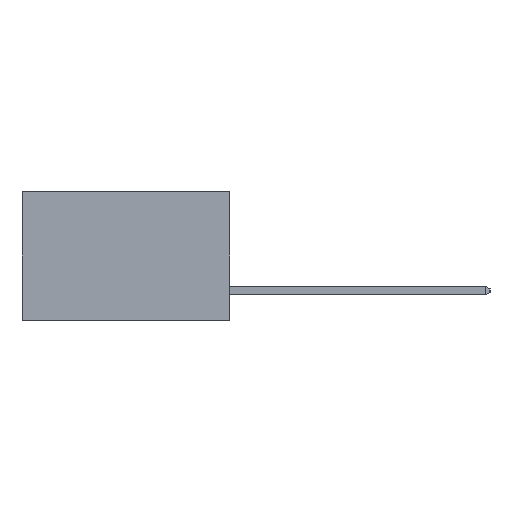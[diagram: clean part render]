
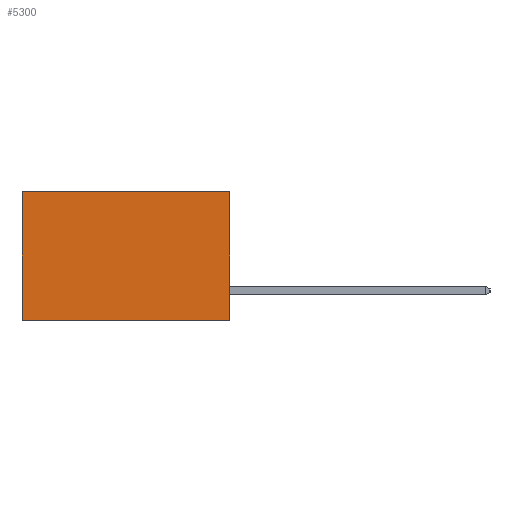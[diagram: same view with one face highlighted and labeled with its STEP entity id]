
A CAD part, left-side view. The second image highlights one B-rep face of the part: STEP entity #5300.
In plain terms, the highlighted planar face has unit normal (-1, 0, 0).
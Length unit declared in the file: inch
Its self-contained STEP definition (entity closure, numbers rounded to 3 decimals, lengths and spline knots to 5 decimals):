
#110 = VERTEX_POINT ( 'NONE', #11537 ) ;
#873 = CARTESIAN_POINT ( 'NONE',  ( 0.298, 0., 0. ) ) ;
#1247 = EDGE_CURVE ( 'NONE', #7658, #110, #11859, .T. ) ;
#2541 = EDGE_CURVE ( 'NONE', #7658, #10924, #6286, .T. ) ;
#2732 = VERTEX_POINT ( 'NONE', #8486 ) ;
#3368 = FACE_OUTER_BOUND ( 'NONE', #9098, .T. ) ;
#3498 = PLANE ( 'NONE',  #4127 ) ;
#3576 = VECTOR ( 'NONE', #9642, 39.37008 ) ;
#4127 = AXIS2_PLACEMENT_3D ( 'NONE', #6442, #6781, #6343 ) ;
#4797 = LINE ( 'NONE', #9197, #6641 ) ;
#5300 = ADVANCED_FACE ( 'NONE', ( #3368 ), #3498, .F. ) ;
#6286 = LINE ( 'NONE', #11158, #3576 ) ;
#6343 = DIRECTION ( 'NONE',  ( 0., 0., -1. ) ) ;
#6442 = CARTESIAN_POINT ( 'NONE',  ( 0.298, 0., 0. ) ) ;
#6463 = EDGE_CURVE ( 'NONE', #110, #2732, #9308, .T. ) ;
#6641 = VECTOR ( 'NONE', #10113, 39.37008 ) ;
#6738 = VECTOR ( 'NONE', #11550, 39.37008 ) ;
#6781 = DIRECTION ( 'NONE',  ( 1., 0., 0. ) ) ;
#6891 = VECTOR ( 'NONE', #9306, 39.37008 ) ;
#7658 = VERTEX_POINT ( 'NONE', #11718 ) ;
#8486 = CARTESIAN_POINT ( 'NONE',  ( 0.298, 0.6, -0.37 ) ) ;
#8659 = CARTESIAN_POINT ( 'NONE',  ( 0.298, 0., -0.37 ) ) ;
#9098 = EDGE_LOOP ( 'NONE', ( #10130, #11279, #9930, #10434 ) ) ;
#9114 = CARTESIAN_POINT ( 'NONE',  ( 0.298, 0.6, 0. ) ) ;
#9197 = CARTESIAN_POINT ( 'NONE',  ( 0.298, 0., -0.37 ) ) ;
#9306 = DIRECTION ( 'NONE',  ( 0., 0., -1. ) ) ;
#9308 = LINE ( 'NONE', #9114, #6891 ) ;
#9642 = DIRECTION ( 'NONE',  ( 0., 0., -1. ) ) ;
#9930 = ORIENTED_EDGE ( 'NONE', *, *, #2541, .F. ) ;
#10042 = EDGE_CURVE ( 'NONE', #10924, #2732, #4797, .T. ) ;
#10113 = DIRECTION ( 'NONE',  ( 0., 1., 0. ) ) ;
#10130 = ORIENTED_EDGE ( 'NONE', *, *, #6463, .T. ) ;
#10434 = ORIENTED_EDGE ( 'NONE', *, *, #1247, .T. ) ;
#10924 = VERTEX_POINT ( 'NONE', #8659 ) ;
#11158 = CARTESIAN_POINT ( 'NONE',  ( 0.298, 0., 0. ) ) ;
#11279 = ORIENTED_EDGE ( 'NONE', *, *, #10042, .F. ) ;
#11537 = CARTESIAN_POINT ( 'NONE',  ( 0.298, 0.6, 0. ) ) ;
#11550 = DIRECTION ( 'NONE',  ( 0., 1., 0. ) ) ;
#11718 = CARTESIAN_POINT ( 'NONE',  ( 0.298, 0., 0. ) ) ;
#11859 = LINE ( 'NONE', #873, #6738 ) ;
